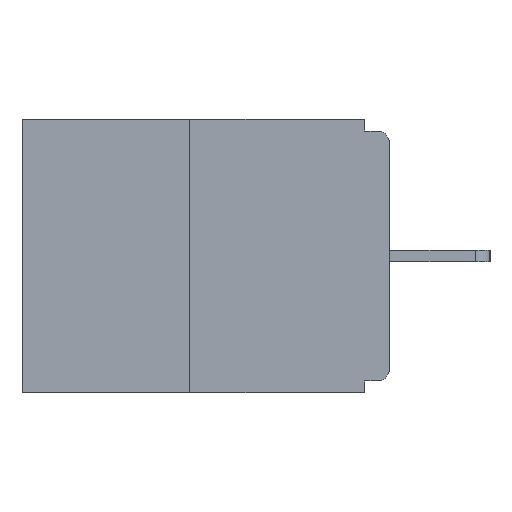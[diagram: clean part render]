
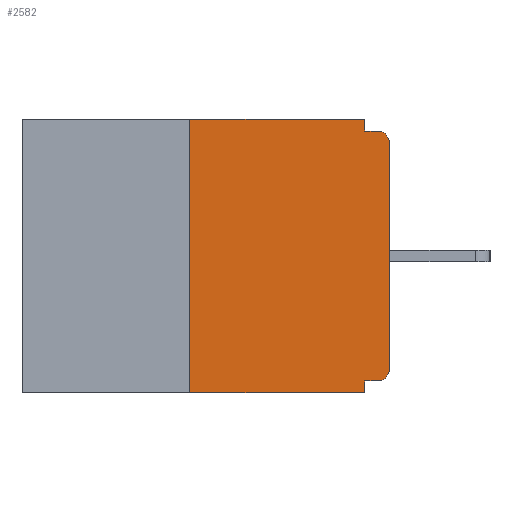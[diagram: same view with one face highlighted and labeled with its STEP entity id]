
A CAD part, left-side view. The second image highlights one B-rep face of the part: STEP entity #2582.
In plain terms, the highlighted planar face has unit normal (-1, 0, 0).
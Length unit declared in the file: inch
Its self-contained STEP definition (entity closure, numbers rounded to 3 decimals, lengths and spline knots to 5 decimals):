
#55 = DIRECTION ( 'NONE',  ( -1., 0., 0. ) ) ;
#114 = CARTESIAN_POINT ( 'NONE',  ( 0., 0.46, -0.343 ) ) ;
#166 = VECTOR ( 'NONE', #9946, 39.37008 ) ;
#189 = EDGE_CURVE ( 'NONE', #6135, #7361, #2468, .T. ) ;
#285 = CARTESIAN_POINT ( 'NONE',  ( 0., 0.031, -0.343 ) ) ;
#384 = CARTESIAN_POINT ( 'NONE',  ( 0., 0.031, -0.328 ) ) ;
#567 = ORIENTED_EDGE ( 'NONE', *, *, #7978, .T. ) ;
#678 = DIRECTION ( 'NONE',  ( -1., 0., 0. ) ) ;
#773 = ORIENTED_EDGE ( 'NONE', *, *, #189, .F. ) ;
#849 = FACE_OUTER_BOUND ( 'NONE', #1045, .T. ) ;
#1045 = EDGE_LOOP ( 'NONE', ( #9087, #9337, #10654, #9565, #10962, #567, #8392, #9070, #773, #3600 ) ) ;
#1105 = VECTOR ( 'NONE', #7614, 39.37008 ) ;
#1135 = EDGE_CURVE ( 'NONE', #1165, #7361, #5567, .T. ) ;
#1165 = VERTEX_POINT ( 'NONE', #5977 ) ;
#1185 = VERTEX_POINT ( 'NONE', #3856 ) ;
#1434 = VECTOR ( 'NONE', #3587, 39.37008 ) ;
#1564 = CARTESIAN_POINT ( 'NONE',  ( 0., 0.015, -0.313 ) ) ;
#1784 = AXIS2_PLACEMENT_3D ( 'NONE', #1564, #678, #3029 ) ;
#1894 = CARTESIAN_POINT ( 'NONE',  ( 0., 0.031, -0.015 ) ) ;
#1950 = EDGE_CURVE ( 'NONE', #10729, #4053, #10175, .T. ) ;
#2184 = AXIS2_PLACEMENT_3D ( 'NONE', #7704, #55, #8645 ) ;
#2435 = DIRECTION ( 'NONE',  ( 0., 0., -1. ) ) ;
#2468 = LINE ( 'NONE', #6779, #1105 ) ;
#2561 = LINE ( 'NONE', #5920, #8903 ) ;
#2582 = ADVANCED_FACE ( 'NONE', ( #849 ), #10315, .F. ) ;
#2973 = EDGE_CURVE ( 'NONE', #4053, #7939, #2561, .T. ) ;
#3029 = DIRECTION ( 'NONE',  ( 0., 0., -1. ) ) ;
#3052 = VECTOR ( 'NONE', #2435, 39.37008 ) ;
#3152 = LINE ( 'NONE', #10838, #166 ) ;
#3468 = DIRECTION ( 'NONE',  ( 1., 0., 0. ) ) ;
#3587 = DIRECTION ( 'NONE',  ( 0., -1., 0. ) ) ;
#3599 = CARTESIAN_POINT ( 'NONE',  ( 0., 0.031, 0. ) ) ;
#3600 = ORIENTED_EDGE ( 'NONE', *, *, #10331, .F. ) ;
#3710 = CARTESIAN_POINT ( 'NONE',  ( 0., 0., 0. ) ) ;
#3830 = VECTOR ( 'NONE', #6638, 39.37008 ) ;
#3856 = CARTESIAN_POINT ( 'NONE',  ( 0., 0., -0.313 ) ) ;
#3961 = VERTEX_POINT ( 'NONE', #8846 ) ;
#4053 = VERTEX_POINT ( 'NONE', #8893 ) ;
#4067 = VECTOR ( 'NONE', #10230, 39.37008 ) ;
#4239 = CARTESIAN_POINT ( 'NONE',  ( 0., 0.46, 0. ) ) ;
#4474 = LINE ( 'NONE', #3710, #6605 ) ;
#4641 = EDGE_CURVE ( 'NONE', #3961, #9907, #10862, .T. ) ;
#5453 = CARTESIAN_POINT ( 'NONE',  ( 0., 0.25, -0.343 ) ) ;
#5567 = CIRCLE ( 'NONE', #2184, 0.015 ) ;
#5745 = VERTEX_POINT ( 'NONE', #285 ) ;
#5920 = CARTESIAN_POINT ( 'NONE',  ( 0., 0.46, 0. ) ) ;
#5934 = DIRECTION ( 'NONE',  ( 0., 0., -1. ) ) ;
#5977 = CARTESIAN_POINT ( 'NONE',  ( 0., 0., -0.03 ) ) ;
#6043 = AXIS2_PLACEMENT_3D ( 'NONE', #4239, #3468, #5934 ) ;
#6135 = VERTEX_POINT ( 'NONE', #1894 ) ;
#6605 = VECTOR ( 'NONE', #7991, 39.37008 ) ;
#6638 = DIRECTION ( 'NONE',  ( 0., 1., 0. ) ) ;
#6691 = CARTESIAN_POINT ( 'NONE',  ( 0., 0., -0.328 ) ) ;
#6779 = CARTESIAN_POINT ( 'NONE',  ( 0., 0., -0.015 ) ) ;
#6839 = CARTESIAN_POINT ( 'NONE',  ( 0., 0.25, 0. ) ) ;
#7361 = VERTEX_POINT ( 'NONE', #10400 ) ;
#7614 = DIRECTION ( 'NONE',  ( 0., -1., 0. ) ) ;
#7695 = EDGE_CURVE ( 'NONE', #9907, #5745, #3152, .T. ) ;
#7704 = CARTESIAN_POINT ( 'NONE',  ( 0., 0.015, -0.03 ) ) ;
#7939 = VERTEX_POINT ( 'NONE', #3599 ) ;
#7946 = EDGE_CURVE ( 'NONE', #1185, #1165, #4474, .T. ) ;
#7978 = EDGE_CURVE ( 'NONE', #3961, #1185, #8560, .T. ) ;
#7991 = DIRECTION ( 'NONE',  ( 0., 0., 1. ) ) ;
#8392 = ORIENTED_EDGE ( 'NONE', *, *, #7946, .T. ) ;
#8544 = LINE ( 'NONE', #114, #1434 ) ;
#8560 = CIRCLE ( 'NONE', #1784, 0.015 ) ;
#8645 = DIRECTION ( 'NONE',  ( 0., 0., -1. ) ) ;
#8846 = CARTESIAN_POINT ( 'NONE',  ( 0., 0.015, -0.328 ) ) ;
#8893 = CARTESIAN_POINT ( 'NONE',  ( 0., 0.25, 0. ) ) ;
#8903 = VECTOR ( 'NONE', #10981, 39.37008 ) ;
#9070 = ORIENTED_EDGE ( 'NONE', *, *, #1135, .T. ) ;
#9087 = ORIENTED_EDGE ( 'NONE', *, *, #2973, .F. ) ;
#9337 = ORIENTED_EDGE ( 'NONE', *, *, #1950, .F. ) ;
#9363 = EDGE_CURVE ( 'NONE', #10729, #5745, #8544, .T. ) ;
#9565 = ORIENTED_EDGE ( 'NONE', *, *, #7695, .F. ) ;
#9907 = VERTEX_POINT ( 'NONE', #384 ) ;
#9946 = DIRECTION ( 'NONE',  ( 0., 0., -1. ) ) ;
#10082 = CARTESIAN_POINT ( 'NONE',  ( 0., 0.031, 0. ) ) ;
#10175 = LINE ( 'NONE', #6839, #4067 ) ;
#10230 = DIRECTION ( 'NONE',  ( 0., 0., 1. ) ) ;
#10315 = PLANE ( 'NONE',  #6043 ) ;
#10331 = EDGE_CURVE ( 'NONE', #7939, #6135, #10971, .T. ) ;
#10400 = CARTESIAN_POINT ( 'NONE',  ( 0., 0.015, -0.015 ) ) ;
#10654 = ORIENTED_EDGE ( 'NONE', *, *, #9363, .T. ) ;
#10729 = VERTEX_POINT ( 'NONE', #5453 ) ;
#10838 = CARTESIAN_POINT ( 'NONE',  ( 0., 0.031, -0.343 ) ) ;
#10862 = LINE ( 'NONE', #6691, #3830 ) ;
#10962 = ORIENTED_EDGE ( 'NONE', *, *, #4641, .F. ) ;
#10971 = LINE ( 'NONE', #10082, #3052 ) ;
#10981 = DIRECTION ( 'NONE',  ( 0., -1., 0. ) ) ;
